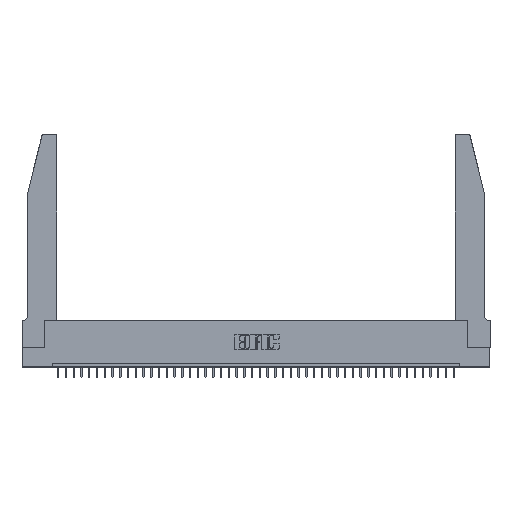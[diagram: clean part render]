
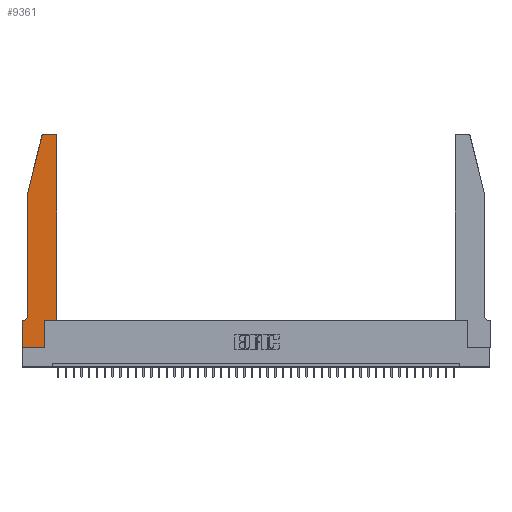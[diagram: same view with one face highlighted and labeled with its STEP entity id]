
A CAD part, top view. The second image highlights one B-rep face of the part: STEP entity #9361.
In plain terms, the highlighted planar face has unit normal (0, 0, 1).
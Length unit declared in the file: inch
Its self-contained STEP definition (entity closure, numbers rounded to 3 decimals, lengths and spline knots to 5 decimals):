
#3 = CARTESIAN_POINT ( 'NONE',  ( 0., 0., 0.37 ) ) ;
#235 = CARTESIAN_POINT ( 'NONE',  ( 0.4505, 2.72, 0.37 ) ) ;
#607 = ORIENTED_EDGE ( 'NONE', *, *, #24791, .T. ) ;
#1790 = CARTESIAN_POINT ( 'NONE',  ( 0.284, 2.72, 0.37 ) ) ;
#2214 = ORIENTED_EDGE ( 'NONE', *, *, #34441, .T. ) ;
#2605 = FACE_OUTER_BOUND ( 'NONE', #12751, .T. ) ;
#2909 = VECTOR ( 'NONE', #36328, 39.37008 ) ;
#3971 = LINE ( 'NONE', #20562, #24174 ) ;
#3979 = DIRECTION ( 'NONE',  ( -1., 0., 0. ) ) ;
#4777 = EDGE_CURVE ( 'NONE', #15475, #9495, #26838, .T. ) ;
#5057 = EDGE_CURVE ( 'NONE', #40452, #42393, #35980, .T. ) ;
#5265 = DIRECTION ( 'NONE',  ( 0., 0., 1. ) ) ;
#5733 = EDGE_CURVE ( 'NONE', #36403, #15475, #27962, .T. ) ;
#6270 = DIRECTION ( 'NONE',  ( 0., -1., 0. ) ) ;
#7017 = EDGE_CURVE ( 'NONE', #41995, #12273, #13168, .T. ) ;
#7128 = DIRECTION ( 'NONE',  ( 0., -1., 0. ) ) ;
#7708 = CARTESIAN_POINT ( 'NONE',  ( 0.4505, 0.35, 0.37 ) ) ;
#7789 = VECTOR ( 'NONE', #31395, 39.37008 ) ;
#8028 = CARTESIAN_POINT ( 'NONE',  ( 0.0755, 2., 0.37 ) ) ;
#8491 = ORIENTED_EDGE ( 'NONE', *, *, #27047, .T. ) ;
#8772 = CARTESIAN_POINT ( 'NONE',  ( 0., 0., 0.37 ) ) ;
#9361 = ADVANCED_FACE ( 'NONE', ( #2605 ), #22429, .T. ) ;
#9495 = VERTEX_POINT ( 'NONE', #235 ) ;
#10408 = VERTEX_POINT ( 'NONE', #17963 ) ;
#11950 = LINE ( 'NONE', #15192, #32617 ) ;
#12060 = EDGE_CURVE ( 'NONE', #12273, #10408, #39517, .T. ) ;
#12235 = VECTOR ( 'NONE', #32045, 39.37008 ) ;
#12273 = VERTEX_POINT ( 'NONE', #27901 ) ;
#12341 = ORIENTED_EDGE ( 'NONE', *, *, #5057, .T. ) ;
#12751 = EDGE_LOOP ( 'NONE', ( #35607, #12341, #8491, #29403, #38756, #29141, #2214, #16654, #607, #14793, #22062, #30678 ) ) ;
#13038 = CARTESIAN_POINT ( 'NONE',  ( 0.4505, 0.35, 0.37 ) ) ;
#13168 = LINE ( 'NONE', #23500, #27325 ) ;
#13908 = DIRECTION ( 'NONE',  ( 1., 0., 0. ) ) ;
#14042 = CIRCLE ( 'NONE', #38140, 0.03 ) ;
#14122 = CARTESIAN_POINT ( 'NONE',  ( 0.4205, 2.72, 0.37 ) ) ;
#14569 = EDGE_CURVE ( 'NONE', #9495, #32002, #14042, .T. ) ;
#14793 = ORIENTED_EDGE ( 'NONE', *, *, #5733, .T. ) ;
#14903 = CARTESIAN_POINT ( 'NONE',  ( 0.2865, 0., 0.37 ) ) ;
#15028 = VERTEX_POINT ( 'NONE', #14903 ) ;
#15192 = CARTESIAN_POINT ( 'NONE',  ( 0.0755, 2., 0.37 ) ) ;
#15475 = VERTEX_POINT ( 'NONE', #13038 ) ;
#15626 = VERTEX_POINT ( 'NONE', #27465 ) ;
#15773 = CARTESIAN_POINT ( 'NONE',  ( 0., 0.35, 0.37 ) ) ;
#15952 = CARTESIAN_POINT ( 'NONE',  ( 0.2605, 2.75, 0.37 ) ) ;
#15987 = DIRECTION ( 'NONE',  ( 0., 0., 1. ) ) ;
#16654 = ORIENTED_EDGE ( 'NONE', *, *, #30817, .T. ) ;
#17183 = VERTEX_POINT ( 'NONE', #24068 ) ;
#17290 = AXIS2_PLACEMENT_3D ( 'NONE', #1790, #5265, #34797 ) ;
#17826 = CARTESIAN_POINT ( 'NONE',  ( 0.2865, 0.35, 0.37 ) ) ;
#17963 = CARTESIAN_POINT ( 'NONE',  ( 0.0055, 0.35, 0.37 ) ) ;
#18589 = EDGE_CURVE ( 'NONE', #32002, #40452, #39009, .T. ) ;
#18753 = VECTOR ( 'NONE', #3979, 39.37008 ) ;
#18794 = LINE ( 'NONE', #3, #28896 ) ;
#19572 = AXIS2_PLACEMENT_3D ( 'NONE', #39772, #23797, #23587 ) ;
#20562 = CARTESIAN_POINT ( 'NONE',  ( 0.2865, 0.35, 0.37 ) ) ;
#22062 = ORIENTED_EDGE ( 'NONE', *, *, #4777, .T. ) ;
#22321 = AXIS2_PLACEMENT_3D ( 'NONE', #15773, #15987, #35606 ) ;
#22332 = LINE ( 'NONE', #8772, #12235 ) ;
#22429 = PLANE ( 'NONE',  #22321 ) ;
#23500 = CARTESIAN_POINT ( 'NONE',  ( 0.0755, 2., 0.37 ) ) ;
#23587 = DIRECTION ( 'NONE',  ( -1., 0., 0. ) ) ;
#23797 = DIRECTION ( 'NONE',  ( 0., 0., -1. ) ) ;
#24001 = DIRECTION ( 'NONE',  ( 0., 1., 0. ) ) ;
#24068 = CARTESIAN_POINT ( 'NONE',  ( 0., 0., 0.37 ) ) ;
#24174 = VECTOR ( 'NONE', #24001, 39.37008 ) ;
#24791 = EDGE_CURVE ( 'NONE', #15028, #36403, #3971, .T. ) ;
#25856 = EDGE_CURVE ( 'NONE', #10408, #15626, #30903, .T. ) ;
#26547 = CARTESIAN_POINT ( 'NONE',  ( 0.25487, 2.72718, 0.37 ) ) ;
#26838 = LINE ( 'NONE', #32673, #2909 ) ;
#27047 = EDGE_CURVE ( 'NONE', #42393, #41995, #11950, .T. ) ;
#27325 = VECTOR ( 'NONE', #7128, 39.37008 ) ;
#27465 = CARTESIAN_POINT ( 'NONE',  ( 0., 0.35, 0.37 ) ) ;
#27901 = CARTESIAN_POINT ( 'NONE',  ( 0.0755, 0.42, 0.37 ) ) ;
#27962 = LINE ( 'NONE', #7708, #7789 ) ;
#28896 = VECTOR ( 'NONE', #6270, 39.37008 ) ;
#29141 = ORIENTED_EDGE ( 'NONE', *, *, #25856, .T. ) ;
#29403 = ORIENTED_EDGE ( 'NONE', *, *, #7017, .T. ) ;
#30678 = ORIENTED_EDGE ( 'NONE', *, *, #14569, .T. ) ;
#30817 = EDGE_CURVE ( 'NONE', #17183, #15028, #22332, .T. ) ;
#30903 = LINE ( 'NONE', #40201, #18753 ) ;
#31395 = DIRECTION ( 'NONE',  ( 1., 0., 0. ) ) ;
#32002 = VERTEX_POINT ( 'NONE', #39689 ) ;
#32045 = DIRECTION ( 'NONE',  ( 1., 0., 0. ) ) ;
#32617 = VECTOR ( 'NONE', #38256, 39.37008 ) ;
#32673 = CARTESIAN_POINT ( 'NONE',  ( 0.4505, 0.35, 0.37 ) ) ;
#33312 = DIRECTION ( 'NONE',  ( 0., 0., 1. ) ) ;
#33880 = CARTESIAN_POINT ( 'NONE',  ( 0.284, 2.75, 0.37 ) ) ;
#34441 = EDGE_CURVE ( 'NONE', #15626, #17183, #18794, .T. ) ;
#34797 = DIRECTION ( 'NONE',  ( 1., 0., 0. ) ) ;
#35606 = DIRECTION ( 'NONE',  ( 1., 0., 0. ) ) ;
#35607 = ORIENTED_EDGE ( 'NONE', *, *, #18589, .T. ) ;
#35980 = CIRCLE ( 'NONE', #17290, 0.03 ) ;
#36328 = DIRECTION ( 'NONE',  ( 0., 1., 0. ) ) ;
#36403 = VERTEX_POINT ( 'NONE', #17826 ) ;
#38140 = AXIS2_PLACEMENT_3D ( 'NONE', #14122, #33312, #13908 ) ;
#38256 = DIRECTION ( 'NONE',  ( -0.239, -0.971, 0. ) ) ;
#38756 = ORIENTED_EDGE ( 'NONE', *, *, #12060, .T. ) ;
#39009 = LINE ( 'NONE', #15952, #42512 ) ;
#39214 = DIRECTION ( 'NONE',  ( -1., 0., 0. ) ) ;
#39517 = CIRCLE ( 'NONE', #19572, 0.07 ) ;
#39689 = CARTESIAN_POINT ( 'NONE',  ( 0.4205, 2.75, 0.37 ) ) ;
#39772 = CARTESIAN_POINT ( 'NONE',  ( 0.0055, 0.42, 0.37 ) ) ;
#40201 = CARTESIAN_POINT ( 'NONE',  ( 0.0755, 0.35, 0.37 ) ) ;
#40452 = VERTEX_POINT ( 'NONE', #33880 ) ;
#41995 = VERTEX_POINT ( 'NONE', #8028 ) ;
#42393 = VERTEX_POINT ( 'NONE', #26547 ) ;
#42512 = VECTOR ( 'NONE', #39214, 39.37008 ) ;
